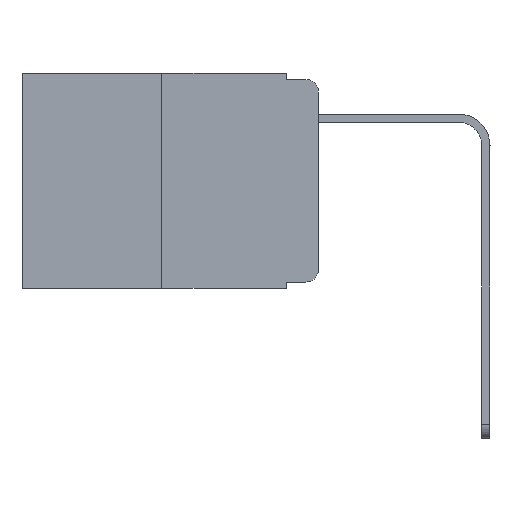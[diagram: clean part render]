
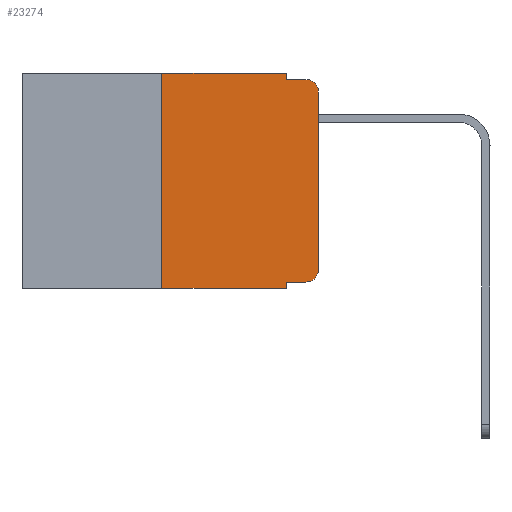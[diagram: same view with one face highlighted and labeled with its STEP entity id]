
A CAD part, left-side view. The second image highlights one B-rep face of the part: STEP entity #23274.
In plain terms, the highlighted planar face has unit normal (-1, 0, 0).
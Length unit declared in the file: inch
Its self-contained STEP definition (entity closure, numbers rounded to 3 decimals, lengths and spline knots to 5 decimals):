
#165 = VERTEX_POINT ( 'NONE', #19866 ) ;
#1364 = DIRECTION ( 'NONE',  ( 0., -1., 0. ) ) ;
#1503 = AXIS2_PLACEMENT_3D ( 'NONE', #7411, #3473, #13114 ) ;
#2053 = ORIENTED_EDGE ( 'NONE', *, *, #16863, .T. ) ;
#2172 = ORIENTED_EDGE ( 'NONE', *, *, #14024, .T. ) ;
#2297 = DIRECTION ( 'NONE',  ( 0., -1., 0. ) ) ;
#3473 = DIRECTION ( 'NONE',  ( -1., 0., 0. ) ) ;
#3799 = EDGE_CURVE ( 'NONE', #13234, #4203, #21640, .T. ) ;
#3941 = CARTESIAN_POINT ( 'NONE',  ( 0., 0.25, -0.343 ) ) ;
#4131 = VERTEX_POINT ( 'NONE', #4300 ) ;
#4203 = VERTEX_POINT ( 'NONE', #18171 ) ;
#4300 = CARTESIAN_POINT ( 'NONE',  ( 0., 0.02, -0.333 ) ) ;
#4350 = CARTESIAN_POINT ( 'NONE',  ( 0., 0.473, 0. ) ) ;
#4405 = ORIENTED_EDGE ( 'NONE', *, *, #9558, .T. ) ;
#4410 = LINE ( 'NONE', #4350, #20894 ) ;
#4710 = CARTESIAN_POINT ( 'NONE',  ( 0., 0.473, 0. ) ) ;
#4951 = CARTESIAN_POINT ( 'NONE',  ( 0., 0.051, -0.01 ) ) ;
#5020 = LINE ( 'NONE', #19514, #19076 ) ;
#5366 = VERTEX_POINT ( 'NONE', #20495 ) ;
#5988 = AXIS2_PLACEMENT_3D ( 'NONE', #4710, #6561, #18258 ) ;
#6498 = DIRECTION ( 'NONE',  ( -1., 0., 0. ) ) ;
#6561 = DIRECTION ( 'NONE',  ( 1., 0., 0. ) ) ;
#6750 = VECTOR ( 'NONE', #9387, 39.37008 ) ;
#6856 = VERTEX_POINT ( 'NONE', #10270 ) ;
#7411 = CARTESIAN_POINT ( 'NONE',  ( 0., 0.02, -0.03 ) ) ;
#7856 = CARTESIAN_POINT ( 'NONE',  ( 0., 0.02, -0.01 ) ) ;
#8063 = DIRECTION ( 'NONE',  ( 0., -1., 0. ) ) ;
#8903 = CIRCLE ( 'NONE', #1503, 0.02 ) ;
#9063 = EDGE_CURVE ( 'NONE', #18646, #13234, #4410, .T. ) ;
#9387 = DIRECTION ( 'NONE',  ( 0., 0., 1. ) ) ;
#9558 = EDGE_CURVE ( 'NONE', #24422, #10932, #8903, .T. ) ;
#10270 = CARTESIAN_POINT ( 'NONE',  ( 0., 0.051, -0.343 ) ) ;
#10741 = PLANE ( 'NONE',  #5988 ) ;
#10845 = EDGE_CURVE ( 'NONE', #15046, #18646, #16341, .T. ) ;
#10932 = VERTEX_POINT ( 'NONE', #7856 ) ;
#11148 = VECTOR ( 'NONE', #12645, 39.37008 ) ;
#11641 = EDGE_CURVE ( 'NONE', #15046, #6856, #16891, .T. ) ;
#11798 = VECTOR ( 'NONE', #2297, 39.37008 ) ;
#11906 = DIRECTION ( 'NONE',  ( 0., -1., 0. ) ) ;
#12062 = VECTOR ( 'NONE', #20111, 39.37008 ) ;
#12488 = CARTESIAN_POINT ( 'NONE',  ( 0., 0., 0. ) ) ;
#12645 = DIRECTION ( 'NONE',  ( 0., 0., 1. ) ) ;
#13114 = DIRECTION ( 'NONE',  ( 0., 0., -1. ) ) ;
#13234 = VERTEX_POINT ( 'NONE', #21711 ) ;
#13396 = VECTOR ( 'NONE', #1364, 39.37008 ) ;
#13421 = AXIS2_PLACEMENT_3D ( 'NONE', #22071, #6498, #21833 ) ;
#13787 = CARTESIAN_POINT ( 'NONE',  ( 0., 0.473, -0.343 ) ) ;
#14024 = EDGE_CURVE ( 'NONE', #5366, #24422, #15040, .T. ) ;
#14591 = ORIENTED_EDGE ( 'NONE', *, *, #3799, .F. ) ;
#14615 = EDGE_CURVE ( 'NONE', #4131, #5366, #17100, .T. ) ;
#15040 = LINE ( 'NONE', #12488, #11148 ) ;
#15046 = VERTEX_POINT ( 'NONE', #3941 ) ;
#15946 = FACE_OUTER_BOUND ( 'NONE', #21103, .T. ) ;
#16116 = CARTESIAN_POINT ( 'NONE',  ( 0., 0.051, 0. ) ) ;
#16341 = LINE ( 'NONE', #18905, #6750 ) ;
#16747 = ORIENTED_EDGE ( 'NONE', *, *, #10845, .F. ) ;
#16797 = ORIENTED_EDGE ( 'NONE', *, *, #24680, .F. ) ;
#16863 = EDGE_CURVE ( 'NONE', #165, #4131, #5020, .T. ) ;
#16891 = LINE ( 'NONE', #13787, #11798 ) ;
#17100 = CIRCLE ( 'NONE', #13421, 0.02 ) ;
#18171 = CARTESIAN_POINT ( 'NONE',  ( 0., 0.051, -0.01 ) ) ;
#18258 = DIRECTION ( 'NONE',  ( 0., 0., -1. ) ) ;
#18646 = VERTEX_POINT ( 'NONE', #21919 ) ;
#18905 = CARTESIAN_POINT ( 'NONE',  ( 0., 0.25, 0. ) ) ;
#19076 = VECTOR ( 'NONE', #8063, 39.37008 ) ;
#19107 = CARTESIAN_POINT ( 'NONE',  ( 0., 0., -0.03 ) ) ;
#19345 = LINE ( 'NONE', #4951, #13396 ) ;
#19514 = CARTESIAN_POINT ( 'NONE',  ( 0., 0.051, -0.333 ) ) ;
#19866 = CARTESIAN_POINT ( 'NONE',  ( 0., 0.051, -0.333 ) ) ;
#20111 = DIRECTION ( 'NONE',  ( 0., 0., -1. ) ) ;
#20495 = CARTESIAN_POINT ( 'NONE',  ( 0., 0., -0.313 ) ) ;
#20894 = VECTOR ( 'NONE', #11906, 39.37008 ) ;
#21103 = EDGE_LOOP ( 'NONE', ( #2172, #4405, #16797, #14591, #22737, #16747, #22729, #24305, #2053, #22711 ) ) ;
#21640 = LINE ( 'NONE', #16116, #22256 ) ;
#21711 = CARTESIAN_POINT ( 'NONE',  ( 0., 0.051, 0. ) ) ;
#21833 = DIRECTION ( 'NONE',  ( 0., 0., -1. ) ) ;
#21919 = CARTESIAN_POINT ( 'NONE',  ( 0., 0.25, 0. ) ) ;
#22071 = CARTESIAN_POINT ( 'NONE',  ( 0., 0.02, -0.313 ) ) ;
#22140 = CARTESIAN_POINT ( 'NONE',  ( 0., 0.051, 0. ) ) ;
#22205 = DIRECTION ( 'NONE',  ( 0., 0., -1. ) ) ;
#22256 = VECTOR ( 'NONE', #22205, 39.37008 ) ;
#22260 = LINE ( 'NONE', #22140, #12062 ) ;
#22711 = ORIENTED_EDGE ( 'NONE', *, *, #14615, .T. ) ;
#22729 = ORIENTED_EDGE ( 'NONE', *, *, #11641, .T. ) ;
#22737 = ORIENTED_EDGE ( 'NONE', *, *, #9063, .F. ) ;
#23227 = EDGE_CURVE ( 'NONE', #165, #6856, #22260, .T. ) ;
#23274 = ADVANCED_FACE ( 'NONE', ( #15946 ), #10741, .F. ) ;
#24305 = ORIENTED_EDGE ( 'NONE', *, *, #23227, .F. ) ;
#24422 = VERTEX_POINT ( 'NONE', #19107 ) ;
#24680 = EDGE_CURVE ( 'NONE', #4203, #10932, #19345, .T. ) ;
